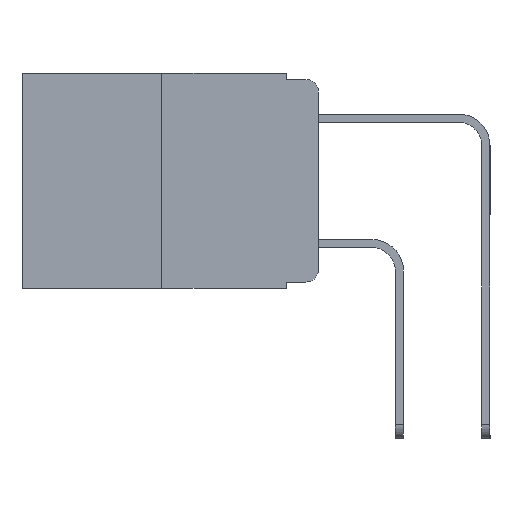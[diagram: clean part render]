
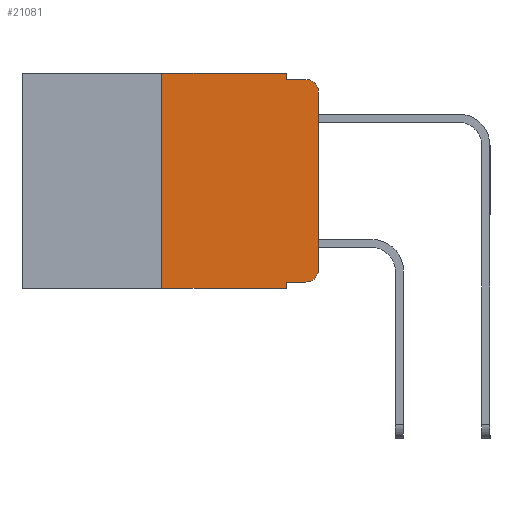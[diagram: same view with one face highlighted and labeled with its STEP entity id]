
A CAD part, left-side view. The second image highlights one B-rep face of the part: STEP entity #21081.
In plain terms, the highlighted planar face has unit normal (-1, 0, 0).
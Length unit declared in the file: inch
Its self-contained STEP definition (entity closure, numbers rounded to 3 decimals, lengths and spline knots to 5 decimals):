
#155 = VECTOR ( 'NONE', #7648, 39.37008 ) ;
#235 = CARTESIAN_POINT ( 'NONE',  ( 0., 0.051, -0.333 ) ) ;
#327 = CARTESIAN_POINT ( 'NONE',  ( 0., 0., -0.03 ) ) ;
#1608 = DIRECTION ( 'NONE',  ( -1., 0., 0. ) ) ;
#2011 = VECTOR ( 'NONE', #2904, 39.37008 ) ;
#2598 = CARTESIAN_POINT ( 'NONE',  ( 0., 0., 0. ) ) ;
#2791 = ORIENTED_EDGE ( 'NONE', *, *, #19106, .T. ) ;
#2904 = DIRECTION ( 'NONE',  ( 0., 0., -1. ) ) ;
#3370 = EDGE_LOOP ( 'NONE', ( #2791, #22633, #8155, #16389, #21794, #10232, #6102, #14934, #18824, #11238 ) ) ;
#3610 = EDGE_CURVE ( 'NONE', #22465, #16793, #7550, .T. ) ;
#3647 = EDGE_CURVE ( 'NONE', #20636, #9738, #17183, .T. ) ;
#3768 = EDGE_CURVE ( 'NONE', #16793, #6224, #9518, .T. ) ;
#3784 = DIRECTION ( 'NONE',  ( 0., 0., -1. ) ) ;
#5161 = LINE ( 'NONE', #18182, #20684 ) ;
#5229 = CARTESIAN_POINT ( 'NONE',  ( 0., 0.25, 0. ) ) ;
#5301 = CARTESIAN_POINT ( 'NONE',  ( 0., 0.051, -0.01 ) ) ;
#5398 = FACE_OUTER_BOUND ( 'NONE', #3370, .T. ) ;
#6102 = ORIENTED_EDGE ( 'NONE', *, *, #15064, .T. ) ;
#6224 = VERTEX_POINT ( 'NONE', #9070 ) ;
#6418 = VECTOR ( 'NONE', #12572, 39.37008 ) ;
#6673 = DIRECTION ( 'NONE',  ( -1., 0., 0. ) ) ;
#6949 = EDGE_CURVE ( 'NONE', #8803, #23248, #7429, .T. ) ;
#6992 = CARTESIAN_POINT ( 'NONE',  ( 0., 0.473, 0. ) ) ;
#7379 = AXIS2_PLACEMENT_3D ( 'NONE', #12538, #1608, #14403 ) ;
#7429 = LINE ( 'NONE', #14679, #12819 ) ;
#7430 = CARTESIAN_POINT ( 'NONE',  ( 0., 0.473, 0. ) ) ;
#7550 = LINE ( 'NONE', #5229, #21370 ) ;
#7648 = DIRECTION ( 'NONE',  ( 0., -1., 0. ) ) ;
#8155 = ORIENTED_EDGE ( 'NONE', *, *, #3647, .F. ) ;
#8412 = AXIS2_PLACEMENT_3D ( 'NONE', #17517, #6673, #19308 ) ;
#8795 = DIRECTION ( 'NONE',  ( 1., 0., 0. ) ) ;
#8803 = VERTEX_POINT ( 'NONE', #12579 ) ;
#9070 = CARTESIAN_POINT ( 'NONE',  ( 0., 0.051, 0. ) ) ;
#9518 = LINE ( 'NONE', #7430, #13798 ) ;
#9738 = VERTEX_POINT ( 'NONE', #13925 ) ;
#9914 = DIRECTION ( 'NONE',  ( 0., 0., 1. ) ) ;
#10232 = ORIENTED_EDGE ( 'NONE', *, *, #3610, .F. ) ;
#10262 = EDGE_CURVE ( 'NONE', #12811, #20105, #15746, .T. ) ;
#10567 = DIRECTION ( 'NONE',  ( 0., 0., 1. ) ) ;
#11021 = LINE ( 'NONE', #235, #155 ) ;
#11238 = ORIENTED_EDGE ( 'NONE', *, *, #10262, .T. ) ;
#11750 = EDGE_CURVE ( 'NONE', #13218, #9738, #22378, .T. ) ;
#12021 = CARTESIAN_POINT ( 'NONE',  ( 0., 0.051, 0. ) ) ;
#12524 = AXIS2_PLACEMENT_3D ( 'NONE', #6992, #8795, #21420 ) ;
#12538 = CARTESIAN_POINT ( 'NONE',  ( 0., 0.02, -0.03 ) ) ;
#12572 = DIRECTION ( 'NONE',  ( 0., -1., 0. ) ) ;
#12579 = CARTESIAN_POINT ( 'NONE',  ( 0., 0.051, -0.333 ) ) ;
#12805 = CARTESIAN_POINT ( 'NONE',  ( 0., 0.051, -0.01 ) ) ;
#12811 = VERTEX_POINT ( 'NONE', #19207 ) ;
#12819 = VECTOR ( 'NONE', #3784, 39.37008 ) ;
#12858 = LINE ( 'NONE', #12021, #2011 ) ;
#12911 = CARTESIAN_POINT ( 'NONE',  ( 0., 0.051, -0.343 ) ) ;
#13218 = VERTEX_POINT ( 'NONE', #327 ) ;
#13467 = VECTOR ( 'NONE', #9914, 39.37008 ) ;
#13798 = VECTOR ( 'NONE', #18273, 39.37008 ) ;
#13925 = CARTESIAN_POINT ( 'NONE',  ( 0., 0.02, -0.01 ) ) ;
#14130 = EDGE_CURVE ( 'NONE', #6224, #20636, #12858, .T. ) ;
#14403 = DIRECTION ( 'NONE',  ( 0., 0., -1. ) ) ;
#14671 = CARTESIAN_POINT ( 'NONE',  ( 0., 0., -0.313 ) ) ;
#14679 = CARTESIAN_POINT ( 'NONE',  ( 0., 0.051, 0. ) ) ;
#14934 = ORIENTED_EDGE ( 'NONE', *, *, #6949, .F. ) ;
#15064 = EDGE_CURVE ( 'NONE', #22465, #23248, #5161, .T. ) ;
#15463 = CARTESIAN_POINT ( 'NONE',  ( 0., 0.25, 0. ) ) ;
#15746 = CIRCLE ( 'NONE', #8412, 0.02 ) ;
#15902 = EDGE_CURVE ( 'NONE', #8803, #12811, #11021, .T. ) ;
#16389 = ORIENTED_EDGE ( 'NONE', *, *, #14130, .F. ) ;
#16793 = VERTEX_POINT ( 'NONE', #15463 ) ;
#17183 = LINE ( 'NONE', #5301, #6418 ) ;
#17517 = CARTESIAN_POINT ( 'NONE',  ( 0., 0.02, -0.313 ) ) ;
#17824 = PLANE ( 'NONE',  #12524 ) ;
#18182 = CARTESIAN_POINT ( 'NONE',  ( 0., 0.473, -0.343 ) ) ;
#18255 = LINE ( 'NONE', #2598, #13467 ) ;
#18273 = DIRECTION ( 'NONE',  ( 0., -1., 0. ) ) ;
#18824 = ORIENTED_EDGE ( 'NONE', *, *, #15902, .T. ) ;
#19106 = EDGE_CURVE ( 'NONE', #20105, #13218, #18255, .T. ) ;
#19207 = CARTESIAN_POINT ( 'NONE',  ( 0., 0.02, -0.333 ) ) ;
#19308 = DIRECTION ( 'NONE',  ( 0., 0., -1. ) ) ;
#19706 = CARTESIAN_POINT ( 'NONE',  ( 0., 0.25, -0.343 ) ) ;
#19978 = DIRECTION ( 'NONE',  ( 0., -1., 0. ) ) ;
#20105 = VERTEX_POINT ( 'NONE', #14671 ) ;
#20636 = VERTEX_POINT ( 'NONE', #12805 ) ;
#20684 = VECTOR ( 'NONE', #19978, 39.37008 ) ;
#21081 = ADVANCED_FACE ( 'NONE', ( #5398 ), #17824, .F. ) ;
#21370 = VECTOR ( 'NONE', #10567, 39.37008 ) ;
#21420 = DIRECTION ( 'NONE',  ( 0., 0., -1. ) ) ;
#21794 = ORIENTED_EDGE ( 'NONE', *, *, #3768, .F. ) ;
#22378 = CIRCLE ( 'NONE', #7379, 0.02 ) ;
#22465 = VERTEX_POINT ( 'NONE', #19706 ) ;
#22633 = ORIENTED_EDGE ( 'NONE', *, *, #11750, .T. ) ;
#23248 = VERTEX_POINT ( 'NONE', #12911 ) ;
